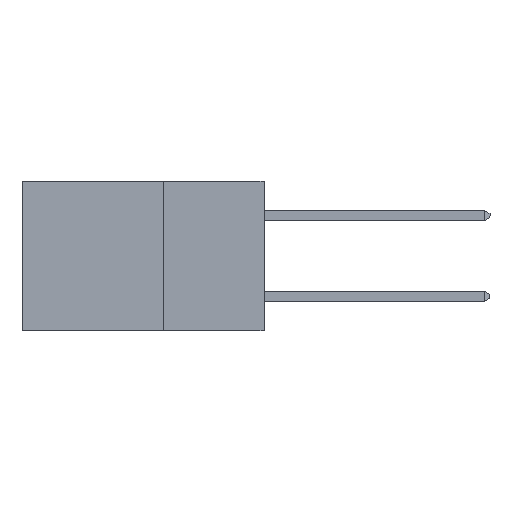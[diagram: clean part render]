
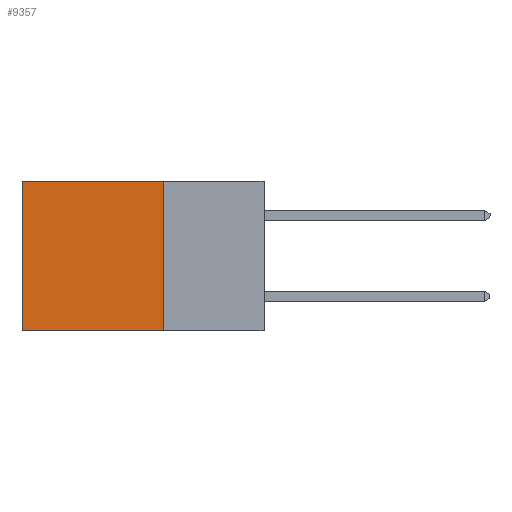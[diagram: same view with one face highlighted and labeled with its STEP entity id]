
A CAD part, left-side view. The second image highlights one B-rep face of the part: STEP entity #9357.
In plain terms, the highlighted planar face has unit normal (-1, 0, 0).
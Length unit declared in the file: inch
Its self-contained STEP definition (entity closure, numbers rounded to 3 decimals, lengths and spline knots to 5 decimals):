
#1950 = VERTEX_POINT ( 'NONE', #18891 ) ;
#3303 = LINE ( 'NONE', #13506, #8898 ) ;
#4448 = VECTOR ( 'NONE', #10570, 39.37008 ) ;
#4474 = VERTEX_POINT ( 'NONE', #15074 ) ;
#5165 = DIRECTION ( 'NONE',  ( 0., 0., -1. ) ) ;
#6420 = CARTESIAN_POINT ( 'NONE',  ( 0.298, 0.25, 0. ) ) ;
#6632 = VECTOR ( 'NONE', #8514, 39.37008 ) ;
#6702 = PLANE ( 'NONE',  #19781 ) ;
#6881 = ORIENTED_EDGE ( 'NONE', *, *, #19563, .T. ) ;
#7566 = EDGE_CURVE ( 'NONE', #17607, #1950, #20221, .T. ) ;
#7634 = VECTOR ( 'NONE', #13482, 39.37008 ) ;
#8514 = DIRECTION ( 'NONE',  ( 0., 0., -1. ) ) ;
#8795 = DIRECTION ( 'NONE',  ( 0., 0., -1. ) ) ;
#8898 = VECTOR ( 'NONE', #5165, 39.37008 ) ;
#9068 = CARTESIAN_POINT ( 'NONE',  ( 0.298, 0.6, -0.37 ) ) ;
#9357 = ADVANCED_FACE ( 'NONE', ( #23611 ), #6702, .F. ) ;
#9649 = CARTESIAN_POINT ( 'NONE',  ( 0.298, 0.25, 0. ) ) ;
#10570 = DIRECTION ( 'NONE',  ( 0., 1., 0. ) ) ;
#11380 = CARTESIAN_POINT ( 'NONE',  ( 0.298, 0.25, -0.37 ) ) ;
#12566 = ORIENTED_EDGE ( 'NONE', *, *, #13615, .F. ) ;
#13139 = LINE ( 'NONE', #11380, #7634 ) ;
#13482 = DIRECTION ( 'NONE',  ( 0., 1., 0. ) ) ;
#13506 = CARTESIAN_POINT ( 'NONE',  ( 0.298, 0.6, 0. ) ) ;
#13615 = EDGE_CURVE ( 'NONE', #17607, #4474, #17626, .T. ) ;
#15074 = CARTESIAN_POINT ( 'NONE',  ( 0.298, 0.25, -0.37 ) ) ;
#17607 = VERTEX_POINT ( 'NONE', #19446 ) ;
#17626 = LINE ( 'NONE', #6420, #6632 ) ;
#18891 = CARTESIAN_POINT ( 'NONE',  ( 0.298, 0.6, 0. ) ) ;
#19446 = CARTESIAN_POINT ( 'NONE',  ( 0.298, 0.25, 0. ) ) ;
#19563 = EDGE_CURVE ( 'NONE', #1950, #24470, #3303, .T. ) ;
#19781 = AXIS2_PLACEMENT_3D ( 'NONE', #23020, #21074, #8795 ) ;
#20221 = LINE ( 'NONE', #9649, #4448 ) ;
#21074 = DIRECTION ( 'NONE',  ( 1., 0., 0. ) ) ;
#21088 = EDGE_LOOP ( 'NONE', ( #6881, #25351, #12566, #21163 ) ) ;
#21163 = ORIENTED_EDGE ( 'NONE', *, *, #7566, .T. ) ;
#23020 = CARTESIAN_POINT ( 'NONE',  ( 0.298, 0.25, 0. ) ) ;
#23611 = FACE_OUTER_BOUND ( 'NONE', #21088, .T. ) ;
#24470 = VERTEX_POINT ( 'NONE', #9068 ) ;
#24536 = EDGE_CURVE ( 'NONE', #4474, #24470, #13139, .T. ) ;
#25351 = ORIENTED_EDGE ( 'NONE', *, *, #24536, .F. ) ;
